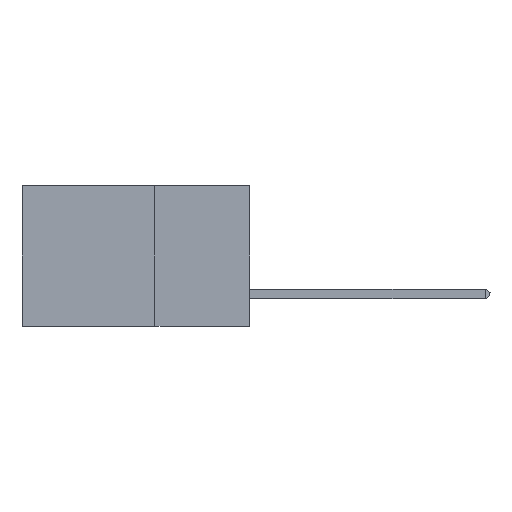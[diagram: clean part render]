
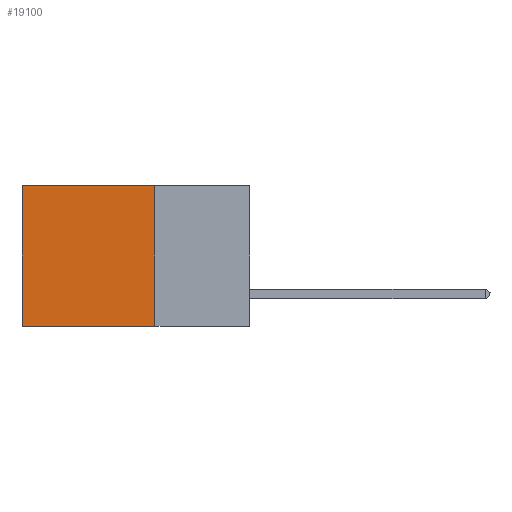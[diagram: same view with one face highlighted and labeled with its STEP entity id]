
A CAD part, left-side view. The second image highlights one B-rep face of the part: STEP entity #19100.
In plain terms, the highlighted planar face has unit normal (-1, 0, 0).
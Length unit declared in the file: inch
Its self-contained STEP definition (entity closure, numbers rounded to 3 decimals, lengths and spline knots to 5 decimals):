
#456 = AXIS2_PLACEMENT_3D ( 'NONE', #19768, #14832, #21871 ) ;
#1203 = CARTESIAN_POINT ( 'NONE',  ( 0.2875, 0.25, -0.37 ) ) ;
#1268 = VECTOR ( 'NONE', #23740, 39.37008 ) ;
#1513 = CARTESIAN_POINT ( 'NONE',  ( 0.2875, 0.25, 0. ) ) ;
#2478 = LINE ( 'NONE', #1203, #10424 ) ;
#2837 = CARTESIAN_POINT ( 'NONE',  ( 0.2875, 0.6, -0.37 ) ) ;
#2877 = LINE ( 'NONE', #5031, #12243 ) ;
#3453 = LINE ( 'NONE', #1513, #1268 ) ;
#5031 = CARTESIAN_POINT ( 'NONE',  ( 0.2875, 0.25, 0. ) ) ;
#5497 = PLANE ( 'NONE',  #456 ) ;
#5892 = ORIENTED_EDGE ( 'NONE', *, *, #7412, .T. ) ;
#6776 = DIRECTION ( 'NONE',  ( 0., 0., -1. ) ) ;
#7086 = ORIENTED_EDGE ( 'NONE', *, *, #17888, .F. ) ;
#7206 = VECTOR ( 'NONE', #6776, 39.37008 ) ;
#7412 = EDGE_CURVE ( 'NONE', #24788, #11206, #2877, .T. ) ;
#7780 = FACE_OUTER_BOUND ( 'NONE', #21034, .T. ) ;
#10424 = VECTOR ( 'NONE', #21255, 39.37008 ) ;
#11206 = VERTEX_POINT ( 'NONE', #28905 ) ;
#11449 = DIRECTION ( 'NONE',  ( 0., 1., 0. ) ) ;
#11644 = ORIENTED_EDGE ( 'NONE', *, *, #20516, .F. ) ;
#12243 = VECTOR ( 'NONE', #11449, 39.37008 ) ;
#14832 = DIRECTION ( 'NONE',  ( 1., 0., 0. ) ) ;
#15994 = CARTESIAN_POINT ( 'NONE',  ( 0.2875, 0.6, 0. ) ) ;
#17888 = EDGE_CURVE ( 'NONE', #23262, #20532, #2478, .T. ) ;
#18031 = ORIENTED_EDGE ( 'NONE', *, *, #27482, .T. ) ;
#18721 = LINE ( 'NONE', #15994, #7206 ) ;
#19100 = ADVANCED_FACE ( 'NONE', ( #7780 ), #5497, .F. ) ;
#19768 = CARTESIAN_POINT ( 'NONE',  ( 0.2875, 0.25, 0. ) ) ;
#20516 = EDGE_CURVE ( 'NONE', #24788, #23262, #3453, .T. ) ;
#20532 = VERTEX_POINT ( 'NONE', #2837 ) ;
#21034 = EDGE_LOOP ( 'NONE', ( #18031, #7086, #11644, #5892 ) ) ;
#21255 = DIRECTION ( 'NONE',  ( 0., 1., 0. ) ) ;
#21871 = DIRECTION ( 'NONE',  ( 0., 0., -1. ) ) ;
#23262 = VERTEX_POINT ( 'NONE', #28297 ) ;
#23740 = DIRECTION ( 'NONE',  ( 0., 0., -1. ) ) ;
#24788 = VERTEX_POINT ( 'NONE', #27140 ) ;
#27140 = CARTESIAN_POINT ( 'NONE',  ( 0.2875, 0.25, 0. ) ) ;
#27482 = EDGE_CURVE ( 'NONE', #11206, #20532, #18721, .T. ) ;
#28297 = CARTESIAN_POINT ( 'NONE',  ( 0.2875, 0.25, -0.37 ) ) ;
#28905 = CARTESIAN_POINT ( 'NONE',  ( 0.2875, 0.6, 0. ) ) ;
